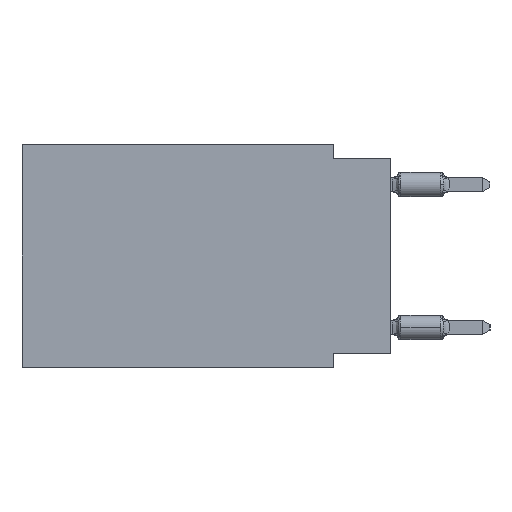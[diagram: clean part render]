
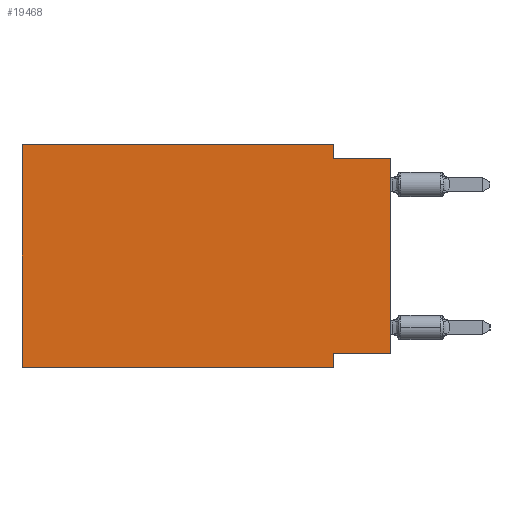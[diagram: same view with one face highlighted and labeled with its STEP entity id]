
A CAD part, left-side view. The second image highlights one B-rep face of the part: STEP entity #19468.
In plain terms, the highlighted planar face has unit normal (-1, 0, 0).
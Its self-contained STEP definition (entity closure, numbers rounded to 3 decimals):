
#264 = VECTOR ( 'NONE', #3081, 1000. ) ;
#326 = DIRECTION ( 'NONE',  ( 0., -1., 0. ) ) ;
#2164 = CARTESIAN_POINT ( 'NONE',  ( 0., 2.54, 0. ) ) ;
#2262 = FACE_OUTER_BOUND ( 'NONE', #26351, .T. ) ;
#2446 = ORIENTED_EDGE ( 'NONE', *, *, #13710, .F. ) ;
#2988 = CARTESIAN_POINT ( 'NONE',  ( 0., 16.383, 0. ) ) ;
#3003 = VERTEX_POINT ( 'NONE', #15445 ) ;
#3081 = DIRECTION ( 'NONE',  ( 0., -1., 0. ) ) ;
#3369 = ORIENTED_EDGE ( 'NONE', *, *, #3798, .T. ) ;
#3701 = EDGE_CURVE ( 'NONE', #6410, #9091, #26686, .T. ) ;
#3773 = CARTESIAN_POINT ( 'NONE',  ( 0., 2.54, -0.635 ) ) ;
#3798 = EDGE_CURVE ( 'NONE', #6410, #24455, #23123, .T. ) ;
#3821 = VECTOR ( 'NONE', #29240, 1000. ) ;
#3883 = CARTESIAN_POINT ( 'NONE',  ( 0., 16.383, 0. ) ) ;
#4308 = CARTESIAN_POINT ( 'NONE',  ( 0., 16.383, 0. ) ) ;
#4821 = VERTEX_POINT ( 'NONE', #3883 ) ;
#5505 = LINE ( 'NONE', #2164, #33133 ) ;
#5893 = LINE ( 'NONE', #31706, #264 ) ;
#6086 = VECTOR ( 'NONE', #23874, 1000. ) ;
#6287 = EDGE_CURVE ( 'NONE', #32732, #4821, #23609, .T. ) ;
#6410 = VERTEX_POINT ( 'NONE', #7301 ) ;
#7301 = CARTESIAN_POINT ( 'NONE',  ( 0., 0., -9.271 ) ) ;
#7869 = VECTOR ( 'NONE', #34360, 1000. ) ;
#8255 = CARTESIAN_POINT ( 'NONE',  ( 0., 2.54, -9.906 ) ) ;
#8380 = EDGE_CURVE ( 'NONE', #9091, #15814, #27429, .T. ) ;
#9091 = VERTEX_POINT ( 'NONE', #22703 ) ;
#12446 = CARTESIAN_POINT ( 'NONE',  ( 0., 0., -9.271 ) ) ;
#13089 = PLANE ( 'NONE',  #28276 ) ;
#13710 = EDGE_CURVE ( 'NONE', #14252, #24455, #5893, .T. ) ;
#14108 = DIRECTION ( 'NONE',  ( 0., 0., -1. ) ) ;
#14252 = VERTEX_POINT ( 'NONE', #3773 ) ;
#15304 = ORIENTED_EDGE ( 'NONE', *, *, #31058, .F. ) ;
#15445 = CARTESIAN_POINT ( 'NONE',  ( 0., 2.54, 0. ) ) ;
#15464 = VECTOR ( 'NONE', #17015, 1000. ) ;
#15626 = DIRECTION ( 'NONE',  ( 0., 0., -1. ) ) ;
#15708 = DIRECTION ( 'NONE',  ( 1., 0., 0. ) ) ;
#15814 = VERTEX_POINT ( 'NONE', #8255 ) ;
#16469 = ORIENTED_EDGE ( 'NONE', *, *, #8380, .F. ) ;
#17015 = DIRECTION ( 'NONE',  ( 0., -1., 0. ) ) ;
#18282 = VECTOR ( 'NONE', #326, 1000. ) ;
#19468 = ADVANCED_FACE ( 'NONE', ( #2262 ), #13089, .F. ) ;
#21787 = CARTESIAN_POINT ( 'NONE',  ( 0., 0., -0.635 ) ) ;
#22703 = CARTESIAN_POINT ( 'NONE',  ( 0., 2.54, -9.271 ) ) ;
#23123 = LINE ( 'NONE', #23478, #7869 ) ;
#23419 = CARTESIAN_POINT ( 'NONE',  ( 0., 16.383, 0. ) ) ;
#23478 = CARTESIAN_POINT ( 'NONE',  ( 0., 0., 0. ) ) ;
#23609 = LINE ( 'NONE', #23419, #3821 ) ;
#23678 = ORIENTED_EDGE ( 'NONE', *, *, #6287, .F. ) ;
#23776 = ORIENTED_EDGE ( 'NONE', *, *, #27966, .F. ) ;
#23874 = DIRECTION ( 'NONE',  ( 0., 1., 0. ) ) ;
#24455 = VERTEX_POINT ( 'NONE', #21787 ) ;
#24516 = DIRECTION ( 'NONE',  ( 0., 0., -1. ) ) ;
#25598 = ORIENTED_EDGE ( 'NONE', *, *, #3701, .F. ) ;
#26351 = EDGE_LOOP ( 'NONE', ( #3369, #2446, #23776, #15304, #23678, #33993, #16469, #25598 ) ) ;
#26686 = LINE ( 'NONE', #12446, #6086 ) ;
#27052 = CARTESIAN_POINT ( 'NONE',  ( 0., 2.54, -9.906 ) ) ;
#27330 = CARTESIAN_POINT ( 'NONE',  ( 0., 16.383, -9.906 ) ) ;
#27429 = LINE ( 'NONE', #27052, #28932 ) ;
#27966 = EDGE_CURVE ( 'NONE', #3003, #14252, #5505, .T. ) ;
#28276 = AXIS2_PLACEMENT_3D ( 'NONE', #4308, #15708, #24516 ) ;
#28932 = VECTOR ( 'NONE', #15626, 1000. ) ;
#29240 = DIRECTION ( 'NONE',  ( 0., 0., 1. ) ) ;
#31058 = EDGE_CURVE ( 'NONE', #4821, #3003, #34239, .T. ) ;
#31706 = CARTESIAN_POINT ( 'NONE',  ( 0., 0., -0.635 ) ) ;
#31932 = LINE ( 'NONE', #32119, #18282 ) ;
#32119 = CARTESIAN_POINT ( 'NONE',  ( 0., 16.383, -9.906 ) ) ;
#32732 = VERTEX_POINT ( 'NONE', #27330 ) ;
#33133 = VECTOR ( 'NONE', #14108, 1000. ) ;
#33993 = ORIENTED_EDGE ( 'NONE', *, *, #34893, .T. ) ;
#34239 = LINE ( 'NONE', #2988, #15464 ) ;
#34360 = DIRECTION ( 'NONE',  ( 0., 0., 1. ) ) ;
#34893 = EDGE_CURVE ( 'NONE', #32732, #15814, #31932, .T. ) ;
